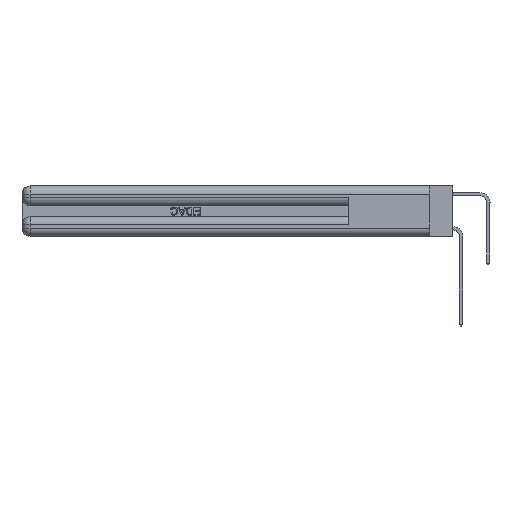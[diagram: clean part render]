
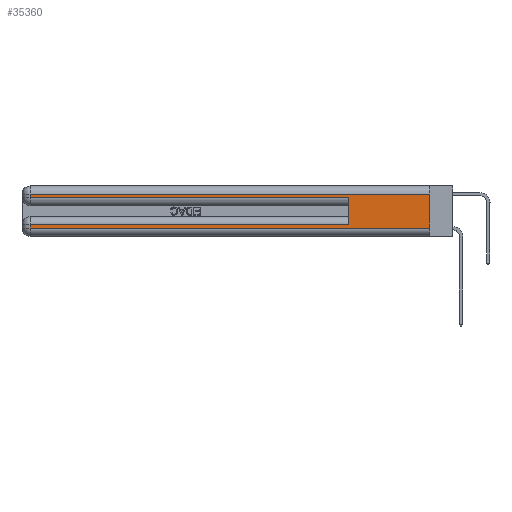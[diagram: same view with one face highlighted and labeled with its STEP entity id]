
A CAD part, left-side view. The second image highlights one B-rep face of the part: STEP entity #35360.
In plain terms, the highlighted planar face has unit normal (-1, 0, 0).
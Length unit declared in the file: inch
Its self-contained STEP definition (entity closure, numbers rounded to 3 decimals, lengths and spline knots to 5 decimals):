
#923 = EDGE_CURVE ( 'NONE', #21677, #31585, #21717, .T. ) ;
#953 = EDGE_CURVE ( 'NONE', #11846, #3857, #28414, .T. ) ;
#1134 = DIRECTION ( 'NONE',  ( 0., 1., 0. ) ) ;
#2251 = CARTESIAN_POINT ( 'NONE',  ( 0., 0., 0.06 ) ) ;
#3697 = VECTOR ( 'NONE', #23118, 39.37008 ) ;
#3736 = CARTESIAN_POINT ( 'NONE',  ( 0., 2.94, 0.285 ) ) ;
#3857 = VERTEX_POINT ( 'NONE', #30163 ) ;
#4355 = EDGE_CURVE ( 'NONE', #7268, #11846, #19326, .T. ) ;
#5157 = VECTOR ( 'NONE', #1134, 39.37008 ) ;
#6761 = LINE ( 'NONE', #12735, #37226 ) ;
#7193 = CARTESIAN_POINT ( 'NONE',  ( 0., 0., 0.31 ) ) ;
#7268 = VERTEX_POINT ( 'NONE', #31662 ) ;
#8230 = ORIENTED_EDGE ( 'NONE', *, *, #953, .T. ) ;
#9491 = ORIENTED_EDGE ( 'NONE', *, *, #14922, .T. ) ;
#9880 = EDGE_CURVE ( 'NONE', #31585, #33237, #31915, .T. ) ;
#10540 = DIRECTION ( 'NONE',  ( 0., -1., 0. ) ) ;
#10671 = DIRECTION ( 'NONE',  ( 0., 0., -1. ) ) ;
#11277 = EDGE_CURVE ( 'NONE', #12497, #33150, #28580, .T. ) ;
#11846 = VERTEX_POINT ( 'NONE', #3736 ) ;
#12497 = VERTEX_POINT ( 'NONE', #7193 ) ;
#12541 = FACE_OUTER_BOUND ( 'NONE', #36660, .T. ) ;
#12735 = CARTESIAN_POINT ( 'NONE',  ( 0., 0., 0.06 ) ) ;
#12828 = VECTOR ( 'NONE', #29604, 39.37008 ) ;
#13347 = CARTESIAN_POINT ( 'NONE',  ( 0., 0., 0.285 ) ) ;
#13453 = DIRECTION ( 'NONE',  ( 0., -1., 0. ) ) ;
#13941 = CARTESIAN_POINT ( 'NONE',  ( 0., 2.94, 0.06 ) ) ;
#14922 = EDGE_CURVE ( 'NONE', #33237, #33150, #6761, .T. ) ;
#15775 = CARTESIAN_POINT ( 'NONE',  ( 0., 0., 0.085 ) ) ;
#17546 = CARTESIAN_POINT ( 'NONE',  ( 0., 2.94, 0.37 ) ) ;
#18080 = ORIENTED_EDGE ( 'NONE', *, *, #20455, .T. ) ;
#18204 = VECTOR ( 'NONE', #10540, 39.37008 ) ;
#18954 = DIRECTION ( 'NONE',  ( 0., 0., 1. ) ) ;
#19326 = LINE ( 'NONE', #17546, #3697 ) ;
#19708 = LINE ( 'NONE', #28448, #32681 ) ;
#20455 = EDGE_CURVE ( 'NONE', #12497, #7268, #19708, .T. ) ;
#21263 = AXIS2_PLACEMENT_3D ( 'NONE', #22243, #22502, #10671 ) ;
#21677 = VERTEX_POINT ( 'NONE', #22302 ) ;
#21717 = LINE ( 'NONE', #15775, #5157 ) ;
#21997 = DIRECTION ( 'NONE',  ( 0., 0., -1. ) ) ;
#22243 = CARTESIAN_POINT ( 'NONE',  ( 0., 0., 0.37 ) ) ;
#22302 = CARTESIAN_POINT ( 'NONE',  ( 0., 0.6, 0.085 ) ) ;
#22502 = DIRECTION ( 'NONE',  ( 1., 0., 0. ) ) ;
#23118 = DIRECTION ( 'NONE',  ( 0., 0., -1. ) ) ;
#24075 = ORIENTED_EDGE ( 'NONE', *, *, #9880, .T. ) ;
#24427 = VECTOR ( 'NONE', #21997, 39.37008 ) ;
#27770 = LINE ( 'NONE', #30518, #32870 ) ;
#28318 = ORIENTED_EDGE ( 'NONE', *, *, #4355, .T. ) ;
#28414 = LINE ( 'NONE', #13347, #18204 ) ;
#28448 = CARTESIAN_POINT ( 'NONE',  ( 0., 0., 0.31 ) ) ;
#28580 = LINE ( 'NONE', #35262, #12828 ) ;
#29604 = DIRECTION ( 'NONE',  ( 0., 0., -1. ) ) ;
#29840 = CARTESIAN_POINT ( 'NONE',  ( 0., 2.94, 0.085 ) ) ;
#29865 = ORIENTED_EDGE ( 'NONE', *, *, #11277, .F. ) ;
#30163 = CARTESIAN_POINT ( 'NONE',  ( 0., 0.6, 0.285 ) ) ;
#30518 = CARTESIAN_POINT ( 'NONE',  ( 0., 0.6, 0.145 ) ) ;
#30702 = CARTESIAN_POINT ( 'NONE',  ( 0., 2.94, 0.37 ) ) ;
#31469 = PLANE ( 'NONE',  #21263 ) ;
#31585 = VERTEX_POINT ( 'NONE', #29840 ) ;
#31662 = CARTESIAN_POINT ( 'NONE',  ( 0., 2.94, 0.31 ) ) ;
#31915 = LINE ( 'NONE', #30702, #24427 ) ;
#32681 = VECTOR ( 'NONE', #37068, 39.37008 ) ;
#32727 = ORIENTED_EDGE ( 'NONE', *, *, #36024, .F. ) ;
#32870 = VECTOR ( 'NONE', #18954, 39.37008 ) ;
#33150 = VERTEX_POINT ( 'NONE', #2251 ) ;
#33237 = VERTEX_POINT ( 'NONE', #13941 ) ;
#35262 = CARTESIAN_POINT ( 'NONE',  ( 0., 0., 0.37 ) ) ;
#35360 = ADVANCED_FACE ( 'NONE', ( #12541 ), #31469, .F. ) ;
#36024 = EDGE_CURVE ( 'NONE', #21677, #3857, #27770, .T. ) ;
#36660 = EDGE_LOOP ( 'NONE', ( #29865, #18080, #28318, #8230, #32727, #37275, #24075, #9491 ) ) ;
#37068 = DIRECTION ( 'NONE',  ( 0., 1., 0. ) ) ;
#37226 = VECTOR ( 'NONE', #13453, 39.37008 ) ;
#37275 = ORIENTED_EDGE ( 'NONE', *, *, #923, .T. ) ;
